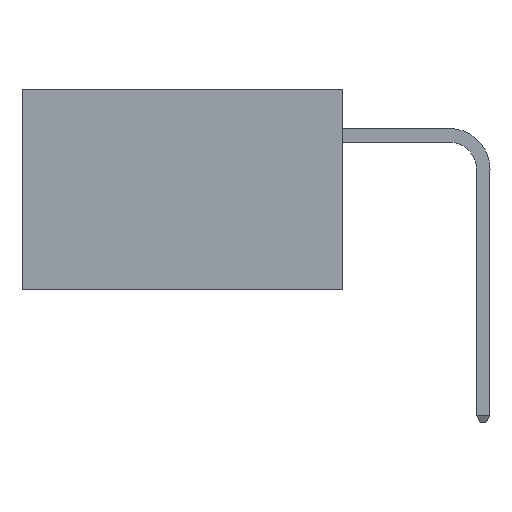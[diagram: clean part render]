
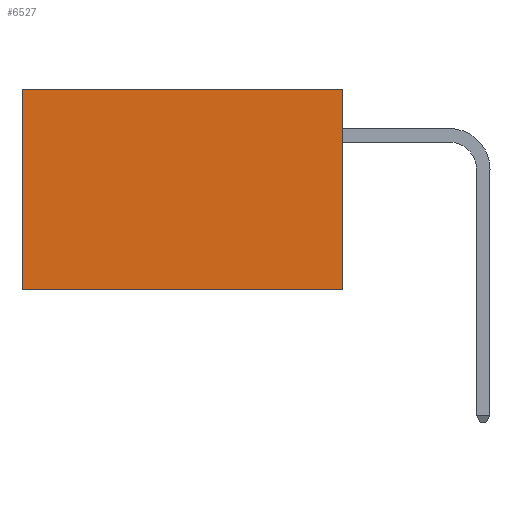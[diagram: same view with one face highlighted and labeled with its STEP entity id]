
A CAD part, left-side view. The second image highlights one B-rep face of the part: STEP entity #6527.
In plain terms, the highlighted planar face has unit normal (-1, 0, 0).
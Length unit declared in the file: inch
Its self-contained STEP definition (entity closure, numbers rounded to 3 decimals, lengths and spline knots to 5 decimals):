
#152 = EDGE_CURVE ( 'NONE', #2588, #5778, #7417, .T. ) ;
#242 = DIRECTION ( 'NONE',  ( 1., 0., 0. ) ) ;
#722 = VECTOR ( 'NONE', #7100, 39.37008 ) ;
#775 = CARTESIAN_POINT ( 'NONE',  ( 0.277, 0.59, -0.37 ) ) ;
#950 = LINE ( 'NONE', #7157, #722 ) ;
#1075 = EDGE_CURVE ( 'NONE', #2266, #2588, #1914, .T. ) ;
#1629 = CARTESIAN_POINT ( 'NONE',  ( 0.277, 0.59, -0.37 ) ) ;
#1914 = LINE ( 'NONE', #8219, #8463 ) ;
#1978 = ORIENTED_EDGE ( 'NONE', *, *, #152, .T. ) ;
#2159 = VECTOR ( 'NONE', #6402, 39.37008 ) ;
#2181 = ORIENTED_EDGE ( 'NONE', *, *, #2702, .F. ) ;
#2240 = AXIS2_PLACEMENT_3D ( 'NONE', #3080, #242, #5229 ) ;
#2266 = VERTEX_POINT ( 'NONE', #3113 ) ;
#2574 = VECTOR ( 'NONE', #7249, 39.37008 ) ;
#2588 = VERTEX_POINT ( 'NONE', #7362 ) ;
#2674 = EDGE_CURVE ( 'NONE', #7294, #5778, #950, .T. ) ;
#2702 = EDGE_CURVE ( 'NONE', #2266, #7294, #7431, .T. ) ;
#3080 = CARTESIAN_POINT ( 'NONE',  ( 0.277, 0., -0.37 ) ) ;
#3113 = CARTESIAN_POINT ( 'NONE',  ( 0.277, 0., 0. ) ) ;
#4398 = CARTESIAN_POINT ( 'NONE',  ( 0.277, 0., -0.37 ) ) ;
#5205 = FACE_OUTER_BOUND ( 'NONE', #7440, .T. ) ;
#5229 = DIRECTION ( 'NONE',  ( 0., 0., -1. ) ) ;
#5778 = VERTEX_POINT ( 'NONE', #1629 ) ;
#6402 = DIRECTION ( 'NONE',  ( 0., 0., -1. ) ) ;
#6435 = CARTESIAN_POINT ( 'NONE',  ( 0.277, 0., -0.37 ) ) ;
#6527 = ADVANCED_FACE ( 'NONE', ( #5205 ), #8127, .F. ) ;
#7100 = DIRECTION ( 'NONE',  ( 0., 1., 0. ) ) ;
#7157 = CARTESIAN_POINT ( 'NONE',  ( 0.277, 0., -0.37 ) ) ;
#7249 = DIRECTION ( 'NONE',  ( 0., 0., -1. ) ) ;
#7286 = ORIENTED_EDGE ( 'NONE', *, *, #2674, .F. ) ;
#7294 = VERTEX_POINT ( 'NONE', #4398 ) ;
#7362 = CARTESIAN_POINT ( 'NONE',  ( 0.277, 0.59, 0. ) ) ;
#7417 = LINE ( 'NONE', #775, #2574 ) ;
#7431 = LINE ( 'NONE', #6435, #2159 ) ;
#7440 = EDGE_LOOP ( 'NONE', ( #1978, #7286, #2181, #7446 ) ) ;
#7446 = ORIENTED_EDGE ( 'NONE', *, *, #1075, .T. ) ;
#8127 = PLANE ( 'NONE',  #2240 ) ;
#8219 = CARTESIAN_POINT ( 'NONE',  ( 0.277, 0., 0. ) ) ;
#8463 = VECTOR ( 'NONE', #8490, 39.37008 ) ;
#8490 = DIRECTION ( 'NONE',  ( 0., 1., 0. ) ) ;
